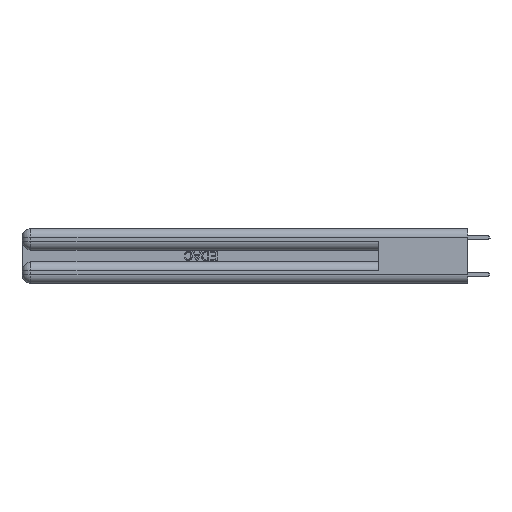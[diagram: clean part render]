
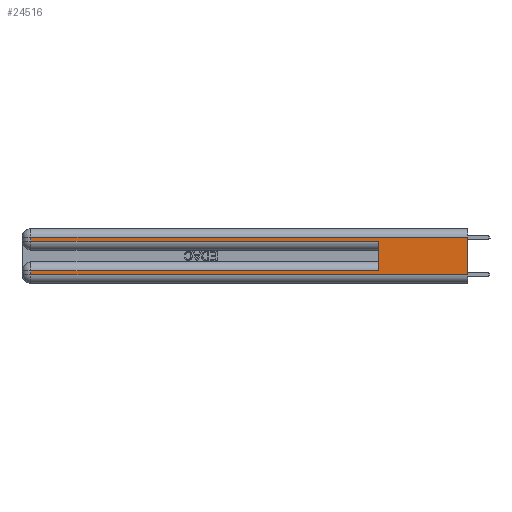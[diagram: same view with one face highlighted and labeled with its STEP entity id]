
A CAD part, left-side view. The second image highlights one B-rep face of the part: STEP entity #24516.
In plain terms, the highlighted planar face has unit normal (-1, 0, 0).
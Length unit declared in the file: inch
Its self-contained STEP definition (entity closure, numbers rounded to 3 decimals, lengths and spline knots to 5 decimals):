
#724 = VECTOR ( 'NONE', #5754, 39.37008 ) ;
#1215 = PLANE ( 'NONE',  #16278 ) ;
#1474 = EDGE_CURVE ( 'NONE', #17869, #14248, #25741, .T. ) ;
#1611 = DIRECTION ( 'NONE',  ( 0., 0., -1. ) ) ;
#2042 = CARTESIAN_POINT ( 'NONE',  ( 0., 0., 0.06 ) ) ;
#2495 = EDGE_CURVE ( 'NONE', #9259, #16302, #20411, .T. ) ;
#3189 = EDGE_CURVE ( 'NONE', #9259, #14248, #14500, .T. ) ;
#4358 = FACE_OUTER_BOUND ( 'NONE', #10257, .T. ) ;
#4773 = DIRECTION ( 'NONE',  ( 0., -1., 0. ) ) ;
#5754 = DIRECTION ( 'NONE',  ( 0., 1., 0. ) ) ;
#5776 = EDGE_CURVE ( 'NONE', #8892, #24793, #21893, .T. ) ;
#6040 = LINE ( 'NONE', #26331, #17486 ) ;
#6848 = VECTOR ( 'NONE', #8797, 39.37008 ) ;
#6972 = CARTESIAN_POINT ( 'NONE',  ( 0., 0., 0.31 ) ) ;
#7099 = CARTESIAN_POINT ( 'NONE',  ( 0., 0., 0.06 ) ) ;
#8146 = ORIENTED_EDGE ( 'NONE', *, *, #23595, .F. ) ;
#8377 = CARTESIAN_POINT ( 'NONE',  ( 0., 0., 0.37 ) ) ;
#8396 = CARTESIAN_POINT ( 'NONE',  ( 0., 0., 0.31 ) ) ;
#8797 = DIRECTION ( 'NONE',  ( 0., 0., -1. ) ) ;
#8892 = VERTEX_POINT ( 'NONE', #28387 ) ;
#9259 = VERTEX_POINT ( 'NONE', #21608 ) ;
#9439 = VECTOR ( 'NONE', #18951, 39.37008 ) ;
#9877 = CARTESIAN_POINT ( 'NONE',  ( 0., 2.94, 0.31 ) ) ;
#10144 = CARTESIAN_POINT ( 'NONE',  ( 0., 2.94, 0.085 ) ) ;
#10257 = EDGE_LOOP ( 'NONE', ( #8146, #14506, #10512, #26661, #20036, #13001, #21079, #27522 ) ) ;
#10263 = VECTOR ( 'NONE', #23054, 39.37008 ) ;
#10512 = ORIENTED_EDGE ( 'NONE', *, *, #25922, .T. ) ;
#10600 = DIRECTION ( 'NONE',  ( 0., 0., -1. ) ) ;
#13001 = ORIENTED_EDGE ( 'NONE', *, *, #2495, .T. ) ;
#14248 = VERTEX_POINT ( 'NONE', #24585 ) ;
#14500 = LINE ( 'NONE', #25272, #26972 ) ;
#14506 = ORIENTED_EDGE ( 'NONE', *, *, #16999, .T. ) ;
#14548 = VERTEX_POINT ( 'NONE', #9877 ) ;
#14551 = LINE ( 'NONE', #8396, #15993 ) ;
#15251 = CARTESIAN_POINT ( 'NONE',  ( 0., 0., 0.085 ) ) ;
#15993 = VECTOR ( 'NONE', #26355, 39.37008 ) ;
#16278 = AXIS2_PLACEMENT_3D ( 'NONE', #21907, #24462, #1611 ) ;
#16302 = VERTEX_POINT ( 'NONE', #10144 ) ;
#16999 = EDGE_CURVE ( 'NONE', #19626, #14548, #14551, .T. ) ;
#17486 = VECTOR ( 'NONE', #10600, 39.37008 ) ;
#17869 = VERTEX_POINT ( 'NONE', #17910 ) ;
#17910 = CARTESIAN_POINT ( 'NONE',  ( 0., 2.94, 0.285 ) ) ;
#18564 = CARTESIAN_POINT ( 'NONE',  ( 0., 0., 0.285 ) ) ;
#18951 = DIRECTION ( 'NONE',  ( 0., -1., 0. ) ) ;
#19626 = VERTEX_POINT ( 'NONE', #6972 ) ;
#20036 = ORIENTED_EDGE ( 'NONE', *, *, #3189, .F. ) ;
#20411 = LINE ( 'NONE', #15251, #724 ) ;
#21079 = ORIENTED_EDGE ( 'NONE', *, *, #27407, .T. ) ;
#21608 = CARTESIAN_POINT ( 'NONE',  ( 0., 0.6, 0.085 ) ) ;
#21882 = VECTOR ( 'NONE', #4773, 39.37008 ) ;
#21893 = LINE ( 'NONE', #2042, #9439 ) ;
#21907 = CARTESIAN_POINT ( 'NONE',  ( 0., 0., 0.37 ) ) ;
#22927 = LINE ( 'NONE', #8377, #6848 ) ;
#23054 = DIRECTION ( 'NONE',  ( 0., 0., -1. ) ) ;
#23595 = EDGE_CURVE ( 'NONE', #19626, #24793, #22927, .T. ) ;
#24462 = DIRECTION ( 'NONE',  ( 1., 0., 0. ) ) ;
#24516 = ADVANCED_FACE ( 'NONE', ( #4358 ), #1215, .F. ) ;
#24585 = CARTESIAN_POINT ( 'NONE',  ( 0., 0.6, 0.285 ) ) ;
#24793 = VERTEX_POINT ( 'NONE', #7099 ) ;
#25175 = DIRECTION ( 'NONE',  ( 0., 0., 1. ) ) ;
#25272 = CARTESIAN_POINT ( 'NONE',  ( 0., 0.6, 0.145 ) ) ;
#25741 = LINE ( 'NONE', #18564, #21882 ) ;
#25922 = EDGE_CURVE ( 'NONE', #14548, #17869, #6040, .T. ) ;
#26331 = CARTESIAN_POINT ( 'NONE',  ( 0., 2.94, 0.37 ) ) ;
#26355 = DIRECTION ( 'NONE',  ( 0., 1., 0. ) ) ;
#26661 = ORIENTED_EDGE ( 'NONE', *, *, #1474, .T. ) ;
#26972 = VECTOR ( 'NONE', #25175, 39.37008 ) ;
#27407 = EDGE_CURVE ( 'NONE', #16302, #8892, #28787, .T. ) ;
#27522 = ORIENTED_EDGE ( 'NONE', *, *, #5776, .T. ) ;
#27531 = CARTESIAN_POINT ( 'NONE',  ( 0., 2.94, 0.37 ) ) ;
#28387 = CARTESIAN_POINT ( 'NONE',  ( 0., 2.94, 0.06 ) ) ;
#28787 = LINE ( 'NONE', #27531, #10263 ) ;
